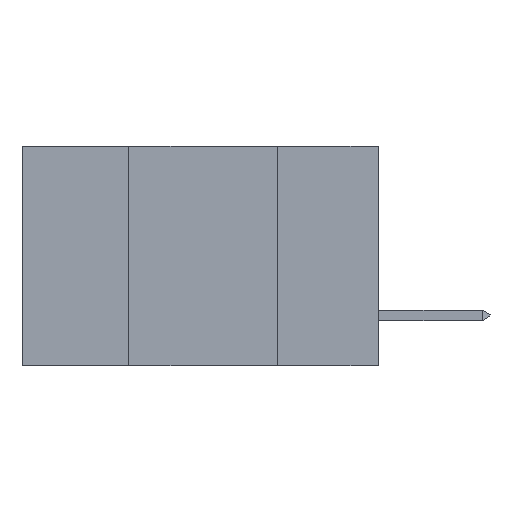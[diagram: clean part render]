
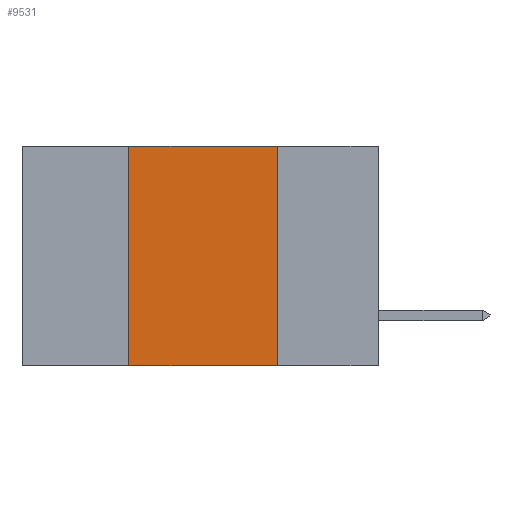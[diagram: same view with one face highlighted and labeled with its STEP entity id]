
A CAD part, left-side view. The second image highlights one B-rep face of the part: STEP entity #9531.
In plain terms, the highlighted planar face has unit normal (-1, 0, 0).
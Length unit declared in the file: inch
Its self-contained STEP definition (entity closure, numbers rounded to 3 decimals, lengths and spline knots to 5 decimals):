
#541 = LINE ( 'NONE', #6381, #1246 ) ;
#625 = AXIS2_PLACEMENT_3D ( 'NONE', #4616, #3924, #6690 ) ;
#630 = LINE ( 'NONE', #1634, #8651 ) ;
#771 = LINE ( 'NONE', #4675, #10911 ) ;
#1054 = DIRECTION ( 'NONE',  ( 0., 0., 1. ) ) ;
#1246 = VECTOR ( 'NONE', #12057, 39.37008 ) ;
#1634 = CARTESIAN_POINT ( 'NONE',  ( 0., 0.6, -0.37 ) ) ;
#1958 = PLANE ( 'NONE',  #625 ) ;
#2447 = DIRECTION ( 'NONE',  ( 0., -1., 0. ) ) ;
#3672 = DIRECTION ( 'NONE',  ( 0., 0., -1. ) ) ;
#3860 = FACE_OUTER_BOUND ( 'NONE', #12286, .T. ) ;
#3924 = DIRECTION ( 'NONE',  ( 1., 0., 0. ) ) ;
#4234 = EDGE_CURVE ( 'NONE', #4911, #11175, #771, .T. ) ;
#4616 = CARTESIAN_POINT ( 'NONE',  ( 0., 0.6, 0. ) ) ;
#4675 = CARTESIAN_POINT ( 'NONE',  ( 0., 0.17, -0.37 ) ) ;
#4911 = VERTEX_POINT ( 'NONE', #7255 ) ;
#5307 = EDGE_CURVE ( 'NONE', #8972, #4911, #541, .T. ) ;
#5712 = ORIENTED_EDGE ( 'NONE', *, *, #5307, .F. ) ;
#6381 = CARTESIAN_POINT ( 'NONE',  ( 0., 0.6, 0. ) ) ;
#6690 = DIRECTION ( 'NONE',  ( 0., 0., -1. ) ) ;
#6859 = CARTESIAN_POINT ( 'NONE',  ( 0., 0.42, 0. ) ) ;
#7255 = CARTESIAN_POINT ( 'NONE',  ( 0., 0.17, 0. ) ) ;
#7736 = LINE ( 'NONE', #10750, #9626 ) ;
#7835 = ORIENTED_EDGE ( 'NONE', *, *, #11630, .T. ) ;
#8125 = EDGE_CURVE ( 'NONE', #8173, #8972, #7736, .T. ) ;
#8173 = VERTEX_POINT ( 'NONE', #9604 ) ;
#8651 = VECTOR ( 'NONE', #2447, 39.37008 ) ;
#8972 = VERTEX_POINT ( 'NONE', #6859 ) ;
#9531 = ADVANCED_FACE ( 'NONE', ( #3860 ), #1958, .F. ) ;
#9604 = CARTESIAN_POINT ( 'NONE',  ( 0., 0.42, -0.37 ) ) ;
#9626 = VECTOR ( 'NONE', #1054, 39.37008 ) ;
#10203 = ORIENTED_EDGE ( 'NONE', *, *, #4234, .F. ) ;
#10750 = CARTESIAN_POINT ( 'NONE',  ( 0., 0.42, -0.37 ) ) ;
#10911 = VECTOR ( 'NONE', #3672, 39.37008 ) ;
#11175 = VERTEX_POINT ( 'NONE', #12099 ) ;
#11630 = EDGE_CURVE ( 'NONE', #8173, #11175, #630, .T. ) ;
#11930 = ORIENTED_EDGE ( 'NONE', *, *, #8125, .F. ) ;
#12057 = DIRECTION ( 'NONE',  ( 0., -1., 0. ) ) ;
#12099 = CARTESIAN_POINT ( 'NONE',  ( 0., 0.17, -0.37 ) ) ;
#12286 = EDGE_LOOP ( 'NONE', ( #10203, #5712, #11930, #7835 ) ) ;
